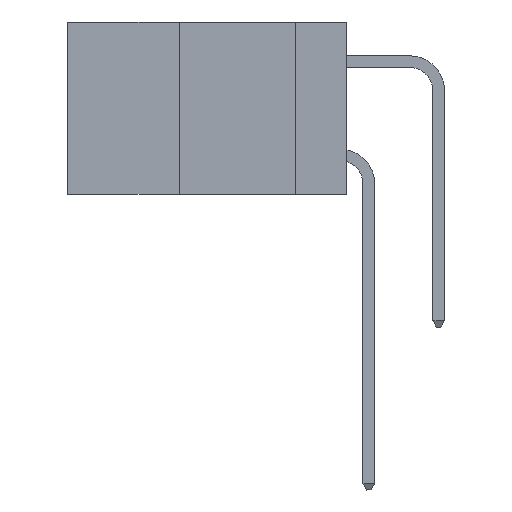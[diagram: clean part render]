
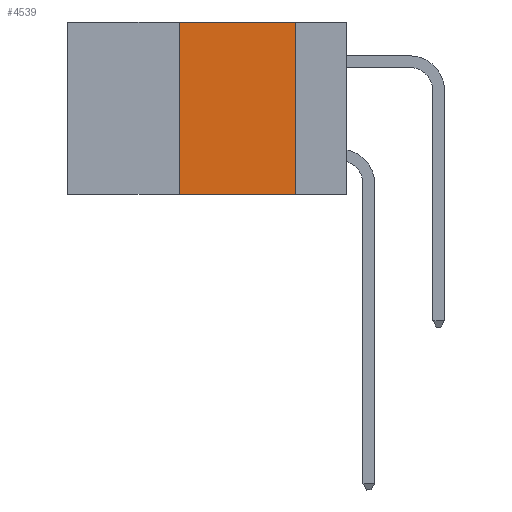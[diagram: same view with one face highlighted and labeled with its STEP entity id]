
A CAD part, left-side view. The second image highlights one B-rep face of the part: STEP entity #4539.
In plain terms, the highlighted planar face has unit normal (-1, 0, 0).
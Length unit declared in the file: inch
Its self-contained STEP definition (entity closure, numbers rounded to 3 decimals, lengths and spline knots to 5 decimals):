
#105 = CARTESIAN_POINT ( 'NONE',  ( 0., 0.36, -0.37 ) ) ;
#804 = EDGE_CURVE ( 'NONE', #4080, #9866, #7951, .T. ) ;
#1110 = CARTESIAN_POINT ( 'NONE',  ( 0., 0.11, 0. ) ) ;
#1289 = CARTESIAN_POINT ( 'NONE',  ( 0., 0.11, 0. ) ) ;
#1385 = CARTESIAN_POINT ( 'NONE',  ( 0., 0.6, 0. ) ) ;
#1744 = CARTESIAN_POINT ( 'NONE',  ( 0., 0.36, 0. ) ) ;
#2117 = DIRECTION ( 'NONE',  ( 0., -1., 0. ) ) ;
#2644 = DIRECTION ( 'NONE',  ( 0., 0., -1. ) ) ;
#3308 = VECTOR ( 'NONE', #2117, 39.37008 ) ;
#3445 = ORIENTED_EDGE ( 'NONE', *, *, #804, .F. ) ;
#4080 = VERTEX_POINT ( 'NONE', #1744 ) ;
#4195 = CARTESIAN_POINT ( 'NONE',  ( 0., 0.6, 0. ) ) ;
#4539 = ADVANCED_FACE ( 'NONE', ( #10612 ), #9577, .F. ) ;
#4774 = CARTESIAN_POINT ( 'NONE',  ( 0., 0.36, 0. ) ) ;
#4846 = VECTOR ( 'NONE', #7854, 39.37008 ) ;
#5191 = VECTOR ( 'NONE', #7127, 39.37008 ) ;
#5363 = VERTEX_POINT ( 'NONE', #13858 ) ;
#5868 = ORIENTED_EDGE ( 'NONE', *, *, #11945, .F. ) ;
#6362 = VERTEX_POINT ( 'NONE', #105 ) ;
#7127 = DIRECTION ( 'NONE',  ( 0., 0., 1. ) ) ;
#7274 = DIRECTION ( 'NONE',  ( 0., 0., -1. ) ) ;
#7369 = ORIENTED_EDGE ( 'NONE', *, *, #9659, .F. ) ;
#7771 = AXIS2_PLACEMENT_3D ( 'NONE', #1385, #14352, #2644 ) ;
#7854 = DIRECTION ( 'NONE',  ( 0., -1., 0. ) ) ;
#7951 = LINE ( 'NONE', #4195, #4846 ) ;
#8996 = LINE ( 'NONE', #15042, #3308 ) ;
#9186 = ORIENTED_EDGE ( 'NONE', *, *, #11368, .T. ) ;
#9577 = PLANE ( 'NONE',  #7771 ) ;
#9659 = EDGE_CURVE ( 'NONE', #6362, #4080, #10908, .T. ) ;
#9866 = VERTEX_POINT ( 'NONE', #1110 ) ;
#10418 = LINE ( 'NONE', #1289, #12459 ) ;
#10612 = FACE_OUTER_BOUND ( 'NONE', #14523, .T. ) ;
#10908 = LINE ( 'NONE', #4774, #5191 ) ;
#11368 = EDGE_CURVE ( 'NONE', #6362, #5363, #8996, .T. ) ;
#11945 = EDGE_CURVE ( 'NONE', #9866, #5363, #10418, .T. ) ;
#12459 = VECTOR ( 'NONE', #7274, 39.37008 ) ;
#13858 = CARTESIAN_POINT ( 'NONE',  ( 0., 0.11, -0.37 ) ) ;
#14352 = DIRECTION ( 'NONE',  ( 1., 0., 0. ) ) ;
#14523 = EDGE_LOOP ( 'NONE', ( #5868, #3445, #7369, #9186 ) ) ;
#15042 = CARTESIAN_POINT ( 'NONE',  ( 0., 0.6, -0.37 ) ) ;
